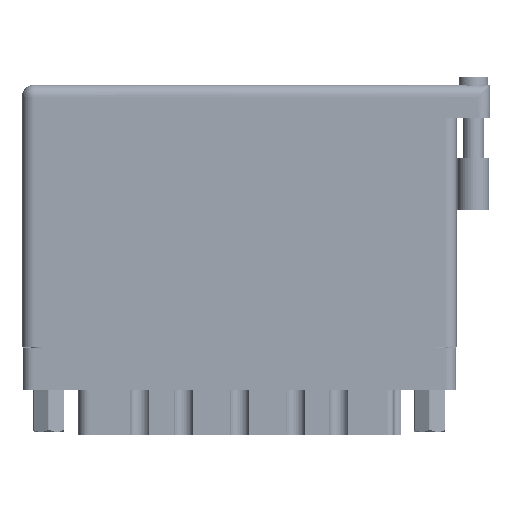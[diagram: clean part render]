
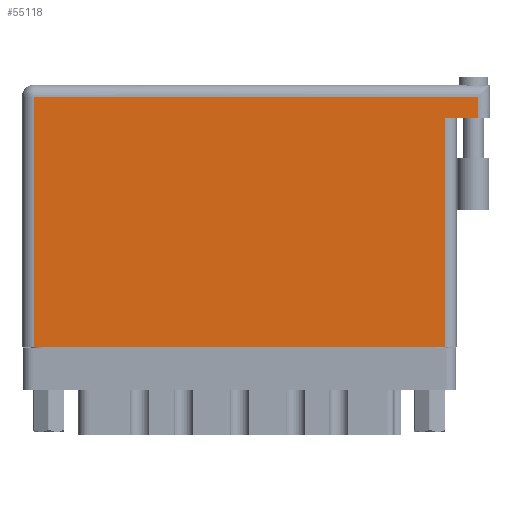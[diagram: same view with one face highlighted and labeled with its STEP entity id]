
A CAD part, front view. The second image highlights one B-rep face of the part: STEP entity #55118.
In plain terms, the highlighted face is planar.
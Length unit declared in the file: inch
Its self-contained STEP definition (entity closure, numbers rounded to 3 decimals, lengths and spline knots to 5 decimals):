
#668 = CARTESIAN_POINT ( 'NONE',  ( 2.73, 1.369, 0. ) ) ;
#1821 = VECTOR ( 'NONE', #4920, 39.37008 ) ;
#2592 = LINE ( 'NONE', #13250, #45413 ) ;
#3903 = CARTESIAN_POINT ( 'NONE',  ( 0., 1.566, 0. ) ) ;
#4920 = DIRECTION ( 'NONE',  ( -1., 0., 0. ) ) ;
#7518 = EDGE_LOOP ( 'NONE', ( #41325, #34158, #45779, #58240, #48845, #42767 ) ) ;
#7909 = DIRECTION ( 'NONE',  ( 0., 0., -1. ) ) ;
#8069 = VECTOR ( 'NONE', #9088, 39.37008 ) ;
#9088 = DIRECTION ( 'NONE',  ( 0., 1., 0. ) ) ;
#9580 = FACE_OUTER_BOUND ( 'NONE', #7518, .T. ) ;
#11166 = VERTEX_POINT ( 'NONE', #60001 ) ;
#11499 = VERTEX_POINT ( 'NONE', #668 ) ;
#12622 = VERTEX_POINT ( 'NONE', #26083 ) ;
#13250 = CARTESIAN_POINT ( 'NONE',  ( 2.73, 1.566, 0. ) ) ;
#15209 = VECTOR ( 'NONE', #51090, 39.37008 ) ;
#17751 = DIRECTION ( 'NONE',  ( -1., 0., 0. ) ) ;
#18745 = CARTESIAN_POINT ( 'NONE',  ( 2.53, 1.369, 0. ) ) ;
#18779 = VECTOR ( 'NONE', #53331, 39.37008 ) ;
#20090 = CARTESIAN_POINT ( 'NONE',  ( 2.73, 1.496, 0. ) ) ;
#21526 = VERTEX_POINT ( 'NONE', #46294 ) ;
#22554 = CARTESIAN_POINT ( 'NONE',  ( 0., 0., 0. ) ) ;
#24968 = LINE ( 'NONE', #22554, #15209 ) ;
#26083 = CARTESIAN_POINT ( 'NONE',  ( 0.07, 0., 0. ) ) ;
#27358 = LINE ( 'NONE', #28191, #1821 ) ;
#28191 = CARTESIAN_POINT ( 'NONE',  ( 0., 1.496, 0. ) ) ;
#30739 = DIRECTION ( 'NONE',  ( 0., -1., 0. ) ) ;
#30747 = LINE ( 'NONE', #58145, #18779 ) ;
#32533 = DIRECTION ( 'NONE',  ( 0., 1., 0. ) ) ;
#33616 = LINE ( 'NONE', #18745, #8069 ) ;
#34158 = ORIENTED_EDGE ( 'NONE', *, *, #51613, .T. ) ;
#34942 = AXIS2_PLACEMENT_3D ( 'NONE', #3903, #7909, #17751 ) ;
#38618 = EDGE_CURVE ( 'NONE', #12622, #11166, #24968, .T. ) ;
#41325 = ORIENTED_EDGE ( 'NONE', *, *, #38618, .T. ) ;
#42750 = EDGE_CURVE ( 'NONE', #44572, #45433, #27358, .T. ) ;
#42767 = ORIENTED_EDGE ( 'NONE', *, *, #52719, .T. ) ;
#44572 = VERTEX_POINT ( 'NONE', #20090 ) ;
#45413 = VECTOR ( 'NONE', #32533, 39.37008 ) ;
#45433 = VERTEX_POINT ( 'NONE', #60670 ) ;
#45779 = ORIENTED_EDGE ( 'NONE', *, *, #60809, .F. ) ;
#46066 = PLANE ( 'NONE',  #34942 ) ;
#46294 = CARTESIAN_POINT ( 'NONE',  ( 2.53, 1.369, 0. ) ) ;
#48845 = ORIENTED_EDGE ( 'NONE', *, *, #42750, .T. ) ;
#50446 = CARTESIAN_POINT ( 'NONE',  ( 0.07, 0., 0. ) ) ;
#51090 = DIRECTION ( 'NONE',  ( 1., 0., 0. ) ) ;
#51613 = EDGE_CURVE ( 'NONE', #11166, #21526, #33616, .T. ) ;
#52719 = EDGE_CURVE ( 'NONE', #45433, #12622, #55945, .T. ) ;
#53331 = DIRECTION ( 'NONE',  ( -1., 0., 0. ) ) ;
#53576 = EDGE_CURVE ( 'NONE', #11499, #44572, #2592, .T. ) ;
#55118 = ADVANCED_FACE ( 'NONE', ( #9580 ), #46066, .F. ) ;
#55945 = LINE ( 'NONE', #50446, #57473 ) ;
#57473 = VECTOR ( 'NONE', #30739, 39.37008 ) ;
#58145 = CARTESIAN_POINT ( 'NONE',  ( 2.8, 1.369, 0. ) ) ;
#58240 = ORIENTED_EDGE ( 'NONE', *, *, #53576, .T. ) ;
#60001 = CARTESIAN_POINT ( 'NONE',  ( 2.53, 0., 0. ) ) ;
#60670 = CARTESIAN_POINT ( 'NONE',  ( 0.07, 1.496, 0. ) ) ;
#60809 = EDGE_CURVE ( 'NONE', #11499, #21526, #30747, .T. ) ;
